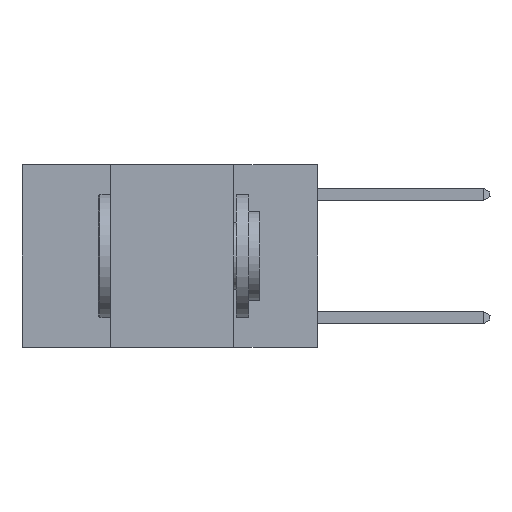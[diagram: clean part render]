
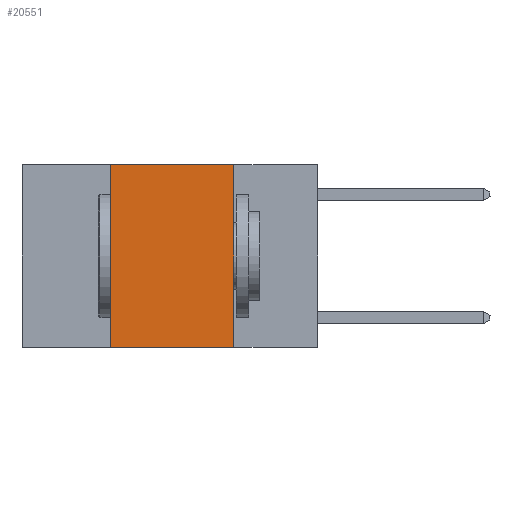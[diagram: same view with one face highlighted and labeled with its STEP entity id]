
A CAD part, left-side view. The second image highlights one B-rep face of the part: STEP entity #20551.
In plain terms, the highlighted planar face has unit normal (-1, 0, 0).
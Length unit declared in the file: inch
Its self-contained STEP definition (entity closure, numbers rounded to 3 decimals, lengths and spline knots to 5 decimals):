
#185 = FACE_OUTER_BOUND ( 'NONE', #18258, .T. ) ;
#861 = ORIENTED_EDGE ( 'NONE', *, *, #19372, .F. ) ;
#3696 = PLANE ( 'NONE',  #9654 ) ;
#4240 = EDGE_CURVE ( 'NONE', #20769, #12039, #6905, .T. ) ;
#4455 = VECTOR ( 'NONE', #14183, 39.37008 ) ;
#4629 = VECTOR ( 'NONE', #11830, 39.37008 ) ;
#5141 = CARTESIAN_POINT ( 'NONE',  ( 0., 0.17, -0.37 ) ) ;
#6792 = CARTESIAN_POINT ( 'NONE',  ( 0., 0.17, 0. ) ) ;
#6905 = LINE ( 'NONE', #6792, #4455 ) ;
#8420 = EDGE_CURVE ( 'NONE', #15100, #20769, #17435, .T. ) ;
#9652 = CARTESIAN_POINT ( 'NONE',  ( 0., 0.17, 0. ) ) ;
#9654 = AXIS2_PLACEMENT_3D ( 'NONE', #14494, #21922, #18381 ) ;
#10363 = ORIENTED_EDGE ( 'NONE', *, *, #8420, .F. ) ;
#11268 = DIRECTION ( 'NONE',  ( 0., -1., 0. ) ) ;
#11694 = CARTESIAN_POINT ( 'NONE',  ( 0., 0.42, -0.37 ) ) ;
#11798 = CARTESIAN_POINT ( 'NONE',  ( 0., 0.42, 0. ) ) ;
#11830 = DIRECTION ( 'NONE',  ( 0., -1., 0. ) ) ;
#12039 = VERTEX_POINT ( 'NONE', #5141 ) ;
#13105 = LINE ( 'NONE', #23162, #15218 ) ;
#13515 = DIRECTION ( 'NONE',  ( 0., 0., 1. ) ) ;
#14183 = DIRECTION ( 'NONE',  ( 0., 0., -1. ) ) ;
#14391 = ORIENTED_EDGE ( 'NONE', *, *, #4240, .F. ) ;
#14494 = CARTESIAN_POINT ( 'NONE',  ( 0., 0.6, 0. ) ) ;
#15100 = VERTEX_POINT ( 'NONE', #19603 ) ;
#15218 = VECTOR ( 'NONE', #11268, 39.37008 ) ;
#15369 = CARTESIAN_POINT ( 'NONE',  ( 0., 0.6, 0. ) ) ;
#15892 = VECTOR ( 'NONE', #13515, 39.37008 ) ;
#17435 = LINE ( 'NONE', #15369, #4629 ) ;
#18258 = EDGE_LOOP ( 'NONE', ( #14391, #10363, #861, #23622 ) ) ;
#18381 = DIRECTION ( 'NONE',  ( 0., 0., -1. ) ) ;
#18966 = LINE ( 'NONE', #11798, #15892 ) ;
#19372 = EDGE_CURVE ( 'NONE', #19397, #15100, #18966, .T. ) ;
#19397 = VERTEX_POINT ( 'NONE', #11694 ) ;
#19603 = CARTESIAN_POINT ( 'NONE',  ( 0., 0.42, 0. ) ) ;
#20551 = ADVANCED_FACE ( 'NONE', ( #185 ), #3696, .F. ) ;
#20769 = VERTEX_POINT ( 'NONE', #9652 ) ;
#21701 = EDGE_CURVE ( 'NONE', #19397, #12039, #13105, .T. ) ;
#21922 = DIRECTION ( 'NONE',  ( 1., 0., 0. ) ) ;
#23162 = CARTESIAN_POINT ( 'NONE',  ( 0., 0.6, -0.37 ) ) ;
#23622 = ORIENTED_EDGE ( 'NONE', *, *, #21701, .T. ) ;
